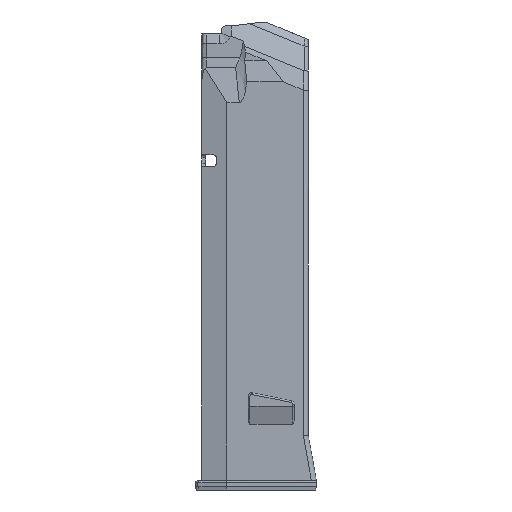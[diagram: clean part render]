
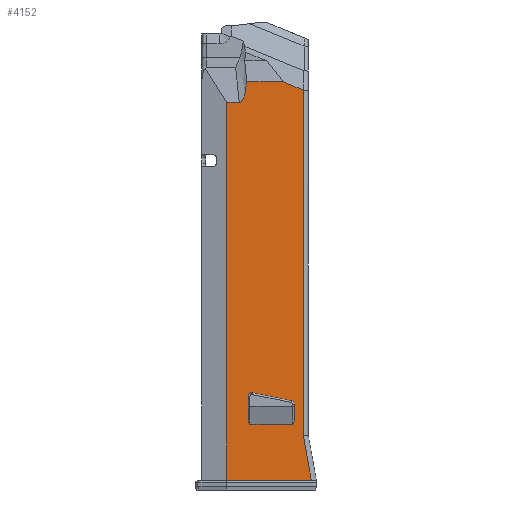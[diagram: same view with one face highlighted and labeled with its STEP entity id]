
A CAD part, left-side view. The second image highlights one B-rep face of the part: STEP entity #4152.
In plain terms, the highlighted planar face has unit normal (-1, 0, 0).
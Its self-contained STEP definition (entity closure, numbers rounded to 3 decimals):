
#191=FACE_BOUND('',#645,.T.);
#252=ELLIPSE('',#4455,1.463,0.503);
#253=ELLIPSE('',#4456,1.005,1.);
#254=ELLIPSE('',#4457,1.005,1.);
#255=ELLIPSE('',#4458,1.463,0.503);
#401=FACE_OUTER_BOUND('',#644,.T.);
#644=EDGE_LOOP('',(#3087,#3088,#3089,#3090,#3091,#3092,#3093,#3094));
#645=EDGE_LOOP('',(#3095,#3096,#3097,#3098,#3099,#3100,#3101,#3102));
#826=LINE('',#5538,#1158);
#832=LINE('',#5561,#1164);
#978=LINE('',#6539,#1310);
#995=LINE('',#6712,#1327);
#998=LINE('',#6751,#1330);
#999=LINE('',#6753,#1331);
#1000=LINE('',#6754,#1332);
#1001=LINE('',#6757,#1333);
#1002=LINE('',#6761,#1334);
#1003=LINE('',#6765,#1335);
#1004=LINE('',#6769,#1336);
#1158=VECTOR('',#4628,10.);
#1164=VECTOR('',#4640,10.043);
#1310=VECTOR('',#4972,10.05);
#1327=VECTOR('',#5023,10.);
#1330=VECTOR('',#5032,10.05);
#1331=VECTOR('',#5033,10.002);
#1332=VECTOR('',#5034,10.);
#1333=VECTOR('',#5035,10.05);
#1334=VECTOR('',#5038,10.);
#1335=VECTOR('',#5041,10.048);
#1336=VECTOR('',#5044,10.);
#1515=B_SPLINE_CURVE_WITH_KNOTS('',3,(#6738,#6739,#6740,#6741,#6742,#6743,
#6744,#6745,#6746,#6747,#6748,#6749,#6750),.UNSPECIFIED.,.F.,.F.,(4,3,3,
3,4),(0.44,0.612,0.907,1.091,
1.202),.UNSPECIFIED.);
#1641=VERTEX_POINT('',#5532);
#1642=VERTEX_POINT('',#5537);
#1648=VERTEX_POINT('',#5560);
#1800=VERTEX_POINT('',#6536);
#1801=VERTEX_POINT('',#6538);
#1826=VERTEX_POINT('',#6711);
#1830=VERTEX_POINT('',#6737);
#1831=VERTEX_POINT('',#6752);
#1832=VERTEX_POINT('',#6755);
#1833=VERTEX_POINT('',#6756);
#1834=VERTEX_POINT('',#6758);
#1835=VERTEX_POINT('',#6760);
#1836=VERTEX_POINT('',#6762);
#1837=VERTEX_POINT('',#6764);
#1838=VERTEX_POINT('',#6766);
#1839=VERTEX_POINT('',#6768);
#2048=EDGE_CURVE('',#1642,#1641,#826,.T.);
#2056=EDGE_CURVE('',#1642,#1648,#832,.T.);
#2267=EDGE_CURVE('',#1800,#1801,#978,.T.);
#2305=EDGE_CURVE('',#1826,#1801,#995,.T.);
#2311=EDGE_CURVE('',#1830,#1641,#1515,.F.);
#2312=EDGE_CURVE('',#1826,#1830,#998,.T.);
#2313=EDGE_CURVE('',#1831,#1800,#999,.T.);
#2314=EDGE_CURVE('',#1648,#1831,#1000,.T.);
#2315=EDGE_CURVE('',#1832,#1833,#1001,.T.);
#2316=EDGE_CURVE('',#1832,#1834,#252,.F.);
#2317=EDGE_CURVE('',#1835,#1834,#1002,.T.);
#2318=EDGE_CURVE('',#1835,#1836,#253,.F.);
#2319=EDGE_CURVE('',#1837,#1836,#1003,.T.);
#2320=EDGE_CURVE('',#1837,#1838,#254,.F.);
#2321=EDGE_CURVE('',#1839,#1838,#1004,.T.);
#2322=EDGE_CURVE('',#1839,#1833,#255,.F.);
#3087=ORIENTED_EDGE('',*,*,#2048,.T.);
#3088=ORIENTED_EDGE('',*,*,#2311,.F.);
#3089=ORIENTED_EDGE('',*,*,#2312,.F.);
#3090=ORIENTED_EDGE('',*,*,#2305,.T.);
#3091=ORIENTED_EDGE('',*,*,#2267,.F.);
#3092=ORIENTED_EDGE('',*,*,#2313,.F.);
#3093=ORIENTED_EDGE('',*,*,#2314,.F.);
#3094=ORIENTED_EDGE('',*,*,#2056,.F.);
#3095=ORIENTED_EDGE('',*,*,#2315,.F.);
#3096=ORIENTED_EDGE('',*,*,#2316,.T.);
#3097=ORIENTED_EDGE('',*,*,#2317,.F.);
#3098=ORIENTED_EDGE('',*,*,#2318,.T.);
#3099=ORIENTED_EDGE('',*,*,#2319,.F.);
#3100=ORIENTED_EDGE('',*,*,#2320,.T.);
#3101=ORIENTED_EDGE('',*,*,#2321,.F.);
#3102=ORIENTED_EDGE('',*,*,#2322,.T.);
#4026=PLANE('',#4454);
#4152=ADVANCED_FACE('',(#401,#191),#4026,.T.);
#4454=AXIS2_PLACEMENT_3D('',#6736,#5030,#5031);
#4455=AXIS2_PLACEMENT_3D('',#6759,#5036,#5037);
#4456=AXIS2_PLACEMENT_3D('',#6763,#5039,#5040);
#4457=AXIS2_PLACEMENT_3D('',#6767,#5042,#5043);
#4458=AXIS2_PLACEMENT_3D('',#6770,#5045,#5046);
#4628=DIRECTION('',(0.,1.,0.));
#4640=DIRECTION('',(0.,-0.925,-0.381));
#4972=DIRECTION('',(0.,1.,0.));
#5023=DIRECTION('',(0.,0.,-1.));
#5030=DIRECTION('center_axis',(-1.,0.,0.));
#5031=DIRECTION('ref_axis',(0.,0.,1.));
#5032=DIRECTION('',(0.,-1.,0.));
#5033=DIRECTION('',(0.,-0.177,-0.984));
#5034=DIRECTION('',(0.,0.,-1.));
#5035=DIRECTION('',(0.,-1.,0.));
#5036=DIRECTION('center_axis',(-1.,0.,0.));
#5037=DIRECTION('ref_axis',(0.,0.,
-1.));
#5038=DIRECTION('',(0.,0.,-1.));
#5039=DIRECTION('center_axis',(-1.,0.,0.));
#5040=DIRECTION('ref_axis',(0.,1.,0.));
#5041=DIRECTION('',(0.,0.98,0.198));
#5042=DIRECTION('center_axis',(-1.,0.,0.));
#5043=DIRECTION('ref_axis',(0.,1.,0.));
#5044=DIRECTION('',(0.,0.,1.));
#5045=DIRECTION('center_axis',(-1.,0.,0.));
#5046=DIRECTION('ref_axis',(0.,0.,-1.));
#5532=CARTESIAN_POINT('',(-10.509,2.449,125.254));
#5537=CARTESIAN_POINT('',(-10.509,-8.781,125.254));
#5538=CARTESIAN_POINT('',(-10.509,-5.828,125.254));
#5560=CARTESIAN_POINT('',(-10.509,-14.905,122.73));
#5561=CARTESIAN_POINT('',(-10.509,-32.689,115.4));
#6536=CARTESIAN_POINT('',(-10.509,-17.349,3.05));
#6538=CARTESIAN_POINT('',(-10.509,8.562,3.05));
#6539=CARTESIAN_POINT('',(-10.509,-8.253,3.05));
#6711=CARTESIAN_POINT('',(-10.509,8.562,118.95));
#6712=CARTESIAN_POINT('',(-10.509,8.562,6.3));
#6736=CARTESIAN_POINT('Origin',(-10.509,-16.413,6.3));
#6737=CARTESIAN_POINT('',(-10.509,4.756,118.95));
#6738=CARTESIAN_POINT('Ctrl Pts',(-10.509,2.449,125.254));
#6739=CARTESIAN_POINT('Ctrl Pts',(-10.509,2.513,124.671));
#6740=CARTESIAN_POINT('Ctrl Pts',(-10.509,2.587,124.084));
#6741=CARTESIAN_POINT('Ctrl Pts',(-10.509,2.683,123.473));
#6742=CARTESIAN_POINT('Ctrl Pts',(-10.509,2.847,122.43));
#6743=CARTESIAN_POINT('Ctrl Pts',(-10.509,3.069,121.378));
#6744=CARTESIAN_POINT('Ctrl Pts',(-10.509,3.372,120.551));
#6745=CARTESIAN_POINT('Ctrl Pts',(-10.509,3.561,120.035));
#6746=CARTESIAN_POINT('Ctrl Pts',(-10.509,3.77,119.598));
#6747=CARTESIAN_POINT('Ctrl Pts',(-10.509,4.077,119.28));
#6748=CARTESIAN_POINT('Ctrl Pts',(-10.509,4.262,119.089));
#6749=CARTESIAN_POINT('Ctrl Pts',(-10.509,4.496,118.95));
#6750=CARTESIAN_POINT('Ctrl Pts',(-10.509,4.756,118.95));
#6751=CARTESIAN_POINT('',(-10.509,-0.081,118.95));
#6752=CARTESIAN_POINT('',(-10.509,-14.905,16.667));
#6753=CARTESIAN_POINT('',(-10.509,-16.47,7.949));
#6754=CARTESIAN_POINT('',(-10.509,-14.905,6.3));
#6755=CARTESIAN_POINT('',(-10.509,1.494,20.2));
#6756=CARTESIAN_POINT('',(-10.509,-11.571,20.2));
#6757=CARTESIAN_POINT('',(-10.509,-14.243,20.2));
#6758=CARTESIAN_POINT('',(-10.509,1.997,21.663));
#6759=CARTESIAN_POINT('Origin',(-10.509,1.494,21.663));
#6760=CARTESIAN_POINT('',(-10.509,1.997,28.824));
#6761=CARTESIAN_POINT('',(-10.509,1.997,13.25));
#6762=CARTESIAN_POINT('',(-10.509,0.792,29.804));
#6763=CARTESIAN_POINT('Origin',(-10.509,0.992,28.824));
#6764=CARTESIAN_POINT('',(-10.509,-11.268,27.363));
#6765=CARTESIAN_POINT('',(-10.509,-9.173,27.787));
#6766=CARTESIAN_POINT('',(-10.509,-12.073,26.383));
#6767=CARTESIAN_POINT('Origin',(-10.509,-11.068,26.383));
#6768=CARTESIAN_POINT('',(-10.509,-12.073,21.663));
#6769=CARTESIAN_POINT('',(-10.509,-12.073,16.75));
#6770=CARTESIAN_POINT('Origin',(-10.509,-11.571,21.663));
